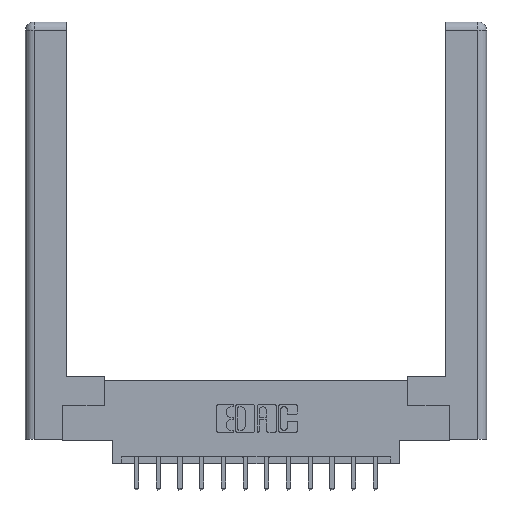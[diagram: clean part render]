
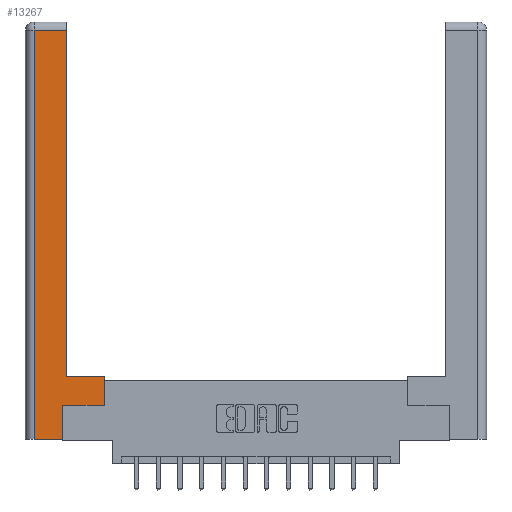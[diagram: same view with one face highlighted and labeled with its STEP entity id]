
A CAD part, top view. The second image highlights one B-rep face of the part: STEP entity #13267.
In plain terms, the highlighted planar face has unit normal (0, 0, 1).
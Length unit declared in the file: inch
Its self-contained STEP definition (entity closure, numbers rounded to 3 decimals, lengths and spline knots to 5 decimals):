
#116 = ORIENTED_EDGE ( 'NONE', *, *, #7514, .T. ) ;
#910 = FACE_OUTER_BOUND ( 'NONE', #2963, .T. ) ;
#929 = VERTEX_POINT ( 'NONE', #14487 ) ;
#931 = CARTESIAN_POINT ( 'NONE',  ( 0.0615, 0., 0. ) ) ;
#1050 = DIRECTION ( 'NONE',  ( 1., 0., 0. ) ) ;
#1123 = EDGE_CURVE ( 'NONE', #2683, #4708, #12743, .T. ) ;
#1167 = CARTESIAN_POINT ( 'NONE',  ( 0.565, 0.245, 0. ) ) ;
#1231 = LINE ( 'NONE', #11048, #12105 ) ;
#1285 = CARTESIAN_POINT ( 'NONE',  ( 0.565, 0.45, 0. ) ) ;
#1521 = LINE ( 'NONE', #15275, #15695 ) ;
#1621 = CARTESIAN_POINT ( 'NONE',  ( 0.265, 0., 0. ) ) ;
#1846 = ORIENTED_EDGE ( 'NONE', *, *, #1123, .T. ) ;
#2041 = VECTOR ( 'NONE', #4656, 39.37008 ) ;
#2254 = EDGE_CURVE ( 'NONE', #14884, #6366, #13862, .T. ) ;
#2683 = VERTEX_POINT ( 'NONE', #4602 ) ;
#2963 = EDGE_LOOP ( 'NONE', ( #7732, #12457, #8882, #14363, #6173, #1846, #4792, #116 ) ) ;
#3096 = EDGE_CURVE ( 'NONE', #3755, #2683, #7238, .T. ) ;
#3111 = CARTESIAN_POINT ( 'NONE',  ( 0., 0., 0. ) ) ;
#3609 = VECTOR ( 'NONE', #7777, 39.37008 ) ;
#3624 = DIRECTION ( 'NONE',  ( -1., 0., 0. ) ) ;
#3755 = VERTEX_POINT ( 'NONE', #15832 ) ;
#3827 = LINE ( 'NONE', #1621, #14106 ) ;
#3986 = LINE ( 'NONE', #11734, #6126 ) ;
#4602 = CARTESIAN_POINT ( 'NONE',  ( 0.265, 0.245, 0. ) ) ;
#4656 = DIRECTION ( 'NONE',  ( 0., -1., 0. ) ) ;
#4708 = VERTEX_POINT ( 'NONE', #6386 ) ;
#4792 = ORIENTED_EDGE ( 'NONE', *, *, #13585, .T. ) ;
#4945 = CARTESIAN_POINT ( 'NONE',  ( 0.0615, 2.94, 0. ) ) ;
#6126 = VECTOR ( 'NONE', #14333, 39.37008 ) ;
#6173 = ORIENTED_EDGE ( 'NONE', *, *, #3096, .T. ) ;
#6304 = VERTEX_POINT ( 'NONE', #1285 ) ;
#6366 = VERTEX_POINT ( 'NONE', #16034 ) ;
#6386 = CARTESIAN_POINT ( 'NONE',  ( 0.565, 0.245, 0. ) ) ;
#6427 = CARTESIAN_POINT ( 'NONE',  ( 0.295, 0.45, 0. ) ) ;
#6625 = VERTEX_POINT ( 'NONE', #11284 ) ;
#6629 = DIRECTION ( 'NONE',  ( 0., 0., -1. ) ) ;
#6815 = DIRECTION ( 'NONE',  ( 0., 1., 0. ) ) ;
#7238 = LINE ( 'NONE', #7954, #11888 ) ;
#7514 = EDGE_CURVE ( 'NONE', #6304, #929, #11552, .T. ) ;
#7732 = ORIENTED_EDGE ( 'NONE', *, *, #11758, .T. ) ;
#7777 = DIRECTION ( 'NONE',  ( -1., 0., 0. ) ) ;
#7954 = CARTESIAN_POINT ( 'NONE',  ( 0.265, 0.245, 0. ) ) ;
#7990 = DIRECTION ( 'NONE',  ( -1., 0., 0. ) ) ;
#8882 = ORIENTED_EDGE ( 'NONE', *, *, #2254, .T. ) ;
#10202 = VECTOR ( 'NONE', #1050, 39.37008 ) ;
#11048 = CARTESIAN_POINT ( 'NONE',  ( 0.0615, 2.94, 0. ) ) ;
#11284 = CARTESIAN_POINT ( 'NONE',  ( 0.295, 2.94, 0. ) ) ;
#11476 = DIRECTION ( 'NONE',  ( 0., 1., 0. ) ) ;
#11552 = LINE ( 'NONE', #6427, #3609 ) ;
#11698 = DIRECTION ( 'NONE',  ( 1., 0., 0. ) ) ;
#11734 = CARTESIAN_POINT ( 'NONE',  ( 0.565, 0.45, 0. ) ) ;
#11758 = EDGE_CURVE ( 'NONE', #929, #6625, #1521, .T. ) ;
#11858 = PLANE ( 'NONE',  #13459 ) ;
#11888 = VECTOR ( 'NONE', #6815, 39.37008 ) ;
#12090 = EDGE_CURVE ( 'NONE', #6366, #3755, #3827, .T. ) ;
#12105 = VECTOR ( 'NONE', #3624, 39.37008 ) ;
#12457 = ORIENTED_EDGE ( 'NONE', *, *, #15172, .T. ) ;
#12743 = LINE ( 'NONE', #1167, #10202 ) ;
#13267 = ADVANCED_FACE ( 'NONE', ( #910 ), #11858, .F. ) ;
#13459 = AXIS2_PLACEMENT_3D ( 'NONE', #3111, #6629, #7990 ) ;
#13585 = EDGE_CURVE ( 'NONE', #4708, #6304, #3986, .T. ) ;
#13862 = LINE ( 'NONE', #931, #2041 ) ;
#14106 = VECTOR ( 'NONE', #11698, 39.37008 ) ;
#14333 = DIRECTION ( 'NONE',  ( 0., 1., 0. ) ) ;
#14363 = ORIENTED_EDGE ( 'NONE', *, *, #12090, .T. ) ;
#14487 = CARTESIAN_POINT ( 'NONE',  ( 0.295, 0.45, 0. ) ) ;
#14884 = VERTEX_POINT ( 'NONE', #4945 ) ;
#15172 = EDGE_CURVE ( 'NONE', #6625, #14884, #1231, .T. ) ;
#15275 = CARTESIAN_POINT ( 'NONE',  ( 0.295, 3., 0. ) ) ;
#15695 = VECTOR ( 'NONE', #11476, 39.37008 ) ;
#15832 = CARTESIAN_POINT ( 'NONE',  ( 0.265, 0., 0. ) ) ;
#16034 = CARTESIAN_POINT ( 'NONE',  ( 0.0615, 0., 0. ) ) ;
